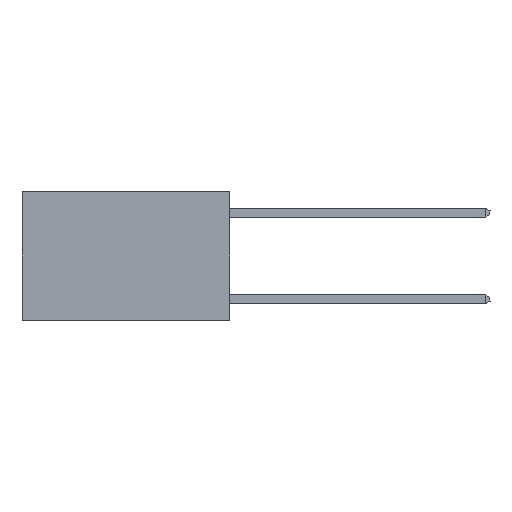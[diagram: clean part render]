
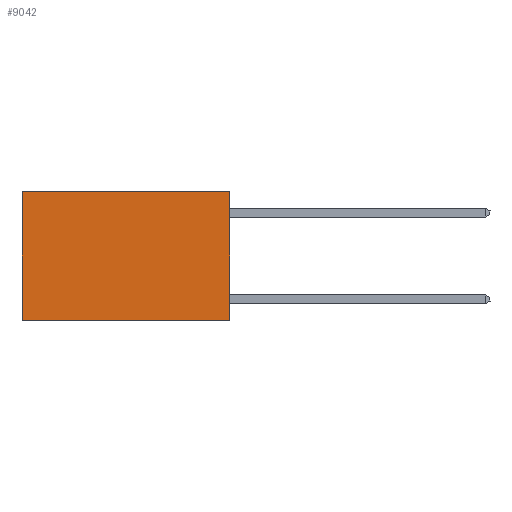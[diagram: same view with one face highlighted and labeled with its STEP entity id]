
A CAD part, left-side view. The second image highlights one B-rep face of the part: STEP entity #9042.
In plain terms, the highlighted planar face has unit normal (-1, 0, 0).
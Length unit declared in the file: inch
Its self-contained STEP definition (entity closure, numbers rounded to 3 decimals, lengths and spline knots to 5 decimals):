
#13 = EDGE_LOOP ( 'NONE', ( #1869, #12931, #4449, #15746 ) ) ;
#117 = EDGE_CURVE ( 'NONE', #7486, #4045, #2169, .T. ) ;
#558 = CARTESIAN_POINT ( 'NONE',  ( 0.2625, 0.6, -0.37 ) ) ;
#657 = DIRECTION ( 'NONE',  ( 1., 0., 0. ) ) ;
#752 = CARTESIAN_POINT ( 'NONE',  ( 0.2625, 0., 0. ) ) ;
#978 = AXIS2_PLACEMENT_3D ( 'NONE', #15883, #657, #14611 ) ;
#1869 = ORIENTED_EDGE ( 'NONE', *, *, #8229, .T. ) ;
#1930 = PLANE ( 'NONE',  #978 ) ;
#2095 = VECTOR ( 'NONE', #6377, 39.37008 ) ;
#2169 = LINE ( 'NONE', #13640, #9334 ) ;
#2442 = CARTESIAN_POINT ( 'NONE',  ( 0.2625, 0., 0. ) ) ;
#2650 = CARTESIAN_POINT ( 'NONE',  ( 0.2625, 0.6, 0. ) ) ;
#3332 = DIRECTION ( 'NONE',  ( 0., 1., 0. ) ) ;
#3459 = EDGE_CURVE ( 'NONE', #13997, #7486, #5926, .T. ) ;
#3754 = CARTESIAN_POINT ( 'NONE',  ( 0.2625, 0.6, 0. ) ) ;
#3954 = VECTOR ( 'NONE', #14782, 39.37008 ) ;
#4045 = VERTEX_POINT ( 'NONE', #558 ) ;
#4449 = ORIENTED_EDGE ( 'NONE', *, *, #3459, .F. ) ;
#5926 = LINE ( 'NONE', #752, #3954 ) ;
#5951 = CARTESIAN_POINT ( 'NONE',  ( 0.2625, 0., -0.37 ) ) ;
#5986 = VERTEX_POINT ( 'NONE', #2650 ) ;
#6377 = DIRECTION ( 'NONE',  ( 0., 0., -1. ) ) ;
#7486 = VERTEX_POINT ( 'NONE', #5951 ) ;
#8229 = EDGE_CURVE ( 'NONE', #5986, #4045, #12907, .T. ) ;
#9042 = ADVANCED_FACE ( 'NONE', ( #13391 ), #1930, .F. ) ;
#9334 = VECTOR ( 'NONE', #12284, 39.37008 ) ;
#10039 = VECTOR ( 'NONE', #3332, 39.37008 ) ;
#12284 = DIRECTION ( 'NONE',  ( 0., 1., 0. ) ) ;
#12907 = LINE ( 'NONE', #3754, #2095 ) ;
#12931 = ORIENTED_EDGE ( 'NONE', *, *, #117, .F. ) ;
#13391 = FACE_OUTER_BOUND ( 'NONE', #13, .T. ) ;
#13640 = CARTESIAN_POINT ( 'NONE',  ( 0.2625, 0., -0.37 ) ) ;
#13948 = LINE ( 'NONE', #16253, #10039 ) ;
#13997 = VERTEX_POINT ( 'NONE', #2442 ) ;
#14611 = DIRECTION ( 'NONE',  ( 0., 0., -1. ) ) ;
#14782 = DIRECTION ( 'NONE',  ( 0., 0., -1. ) ) ;
#15746 = ORIENTED_EDGE ( 'NONE', *, *, #16734, .T. ) ;
#15883 = CARTESIAN_POINT ( 'NONE',  ( 0.2625, 0., 0. ) ) ;
#16253 = CARTESIAN_POINT ( 'NONE',  ( 0.2625, 0., 0. ) ) ;
#16734 = EDGE_CURVE ( 'NONE', #13997, #5986, #13948, .T. ) ;
